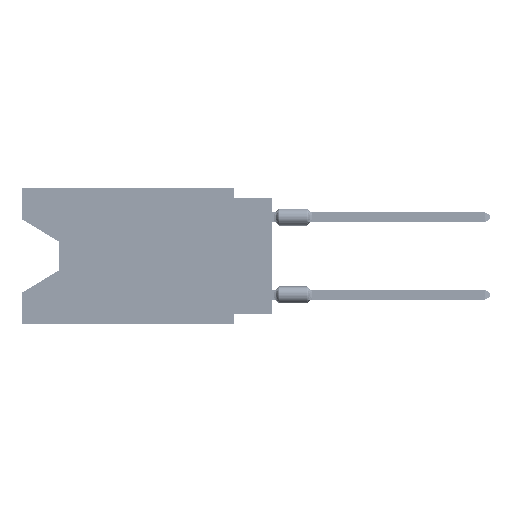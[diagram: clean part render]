
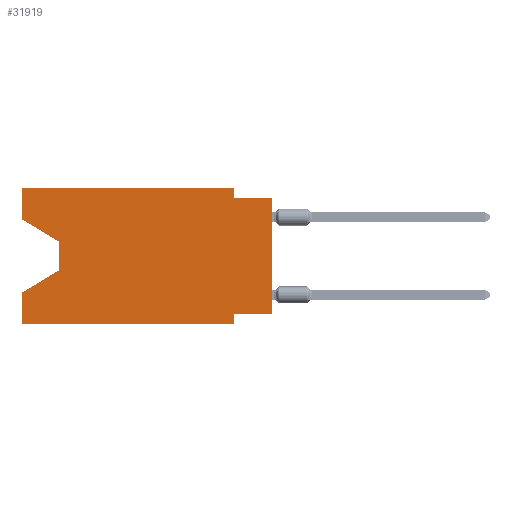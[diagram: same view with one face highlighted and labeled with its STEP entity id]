
A CAD part, left-side view. The second image highlights one B-rep face of the part: STEP entity #31919.
In plain terms, the highlighted planar face has unit normal (-1, 0, 0).
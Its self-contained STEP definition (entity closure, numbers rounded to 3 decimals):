
#1838 = AXIS2_PLACEMENT_3D ( 'NONE', #49395, #35175, #50359 ) ;
#1902 = EDGE_CURVE ( 'NONE', #17807, #44442, #88935, .T. ) ;
#2507 = VECTOR ( 'NONE', #56812, 1000. ) ;
#3308 = CARTESIAN_POINT ( 'NONE',  ( 0., 2.54, 0. ) ) ;
#3503 = VERTEX_POINT ( 'NONE', #51038 ) ;
#3532 = VECTOR ( 'NONE', #49575, 1000. ) ;
#3812 = CARTESIAN_POINT ( 'NONE',  ( 0., 16.383, -2.038 ) ) ;
#4411 = LINE ( 'NONE', #34366, #3532 ) ;
#4842 = VERTEX_POINT ( 'NONE', #69759 ) ;
#5623 = VECTOR ( 'NONE', #85334, 1000. ) ;
#6007 = LINE ( 'NONE', #35966, #92665 ) ;
#7443 = DIRECTION ( 'NONE',  ( 0., 0., -1. ) ) ;
#7530 = EDGE_CURVE ( 'NONE', #15331, #3503, #85624, .T. ) ;
#8111 = DIRECTION ( 'NONE',  ( 0., 0., -1. ) ) ;
#8975 = CARTESIAN_POINT ( 'NONE',  ( 0., 16.383, -6.852 ) ) ;
#10150 = CARTESIAN_POINT ( 'NONE',  ( 0., 0., -0.635 ) ) ;
#10381 = DIRECTION ( 'NONE',  ( 0., 1., 0. ) ) ;
#14312 = DIRECTION ( 'NONE',  ( 0., -1., 0. ) ) ;
#15331 = VERTEX_POINT ( 'NONE', #56127 ) ;
#16073 = VECTOR ( 'NONE', #48302, 1000. ) ;
#17807 = VERTEX_POINT ( 'NONE', #62234 ) ;
#19108 = EDGE_CURVE ( 'NONE', #44442, #82172, #93631, .T. ) ;
#19484 = PLANE ( 'NONE',  #1838 ) ;
#20814 = CARTESIAN_POINT ( 'NONE',  ( 0., 16.383, 0. ) ) ;
#20960 = CARTESIAN_POINT ( 'NONE',  ( 0., 16.383, -2.038 ) ) ;
#21267 = EDGE_LOOP ( 'NONE', ( #82074, #61064, #83660, #91899, #30325, #90696, #51275, #46634, #25352, #51942, #89945, #39362 ) ) ;
#23755 = EDGE_CURVE ( 'NONE', #66748, #15331, #47176, .T. ) ;
#24647 = CARTESIAN_POINT ( 'NONE',  ( 0., 13.97, -5.385 ) ) ;
#25352 = ORIENTED_EDGE ( 'NONE', *, *, #64418, .F. ) ;
#26879 = LINE ( 'NONE', #3812, #2507 ) ;
#28476 = EDGE_CURVE ( 'NONE', #66748, #57467, #29605, .T. ) ;
#28589 = DIRECTION ( 'NONE',  ( 0., 0., 1. ) ) ;
#28646 = VECTOR ( 'NONE', #14312, 1000. ) ;
#28647 = DIRECTION ( 'NONE',  ( 0., 0., 1. ) ) ;
#29263 = EDGE_CURVE ( 'NONE', #83175, #4842, #93589, .T. ) ;
#29605 = LINE ( 'NONE', #52175, #47051 ) ;
#30325 = ORIENTED_EDGE ( 'NONE', *, *, #90097, .T. ) ;
#30608 = CARTESIAN_POINT ( 'NONE',  ( 0., 16.383, 0. ) ) ;
#31919 = ADVANCED_FACE ( 'NONE', ( #48909 ), #19484, .F. ) ;
#34366 = CARTESIAN_POINT ( 'NONE',  ( 0., 16.383, -8.89 ) ) ;
#34486 = VECTOR ( 'NONE', #10381, 1000. ) ;
#35175 = DIRECTION ( 'NONE',  ( 1., 0., 0. ) ) ;
#35966 = CARTESIAN_POINT ( 'NONE',  ( 0., 16.383, 0. ) ) ;
#39065 = VECTOR ( 'NONE', #8111, 1000. ) ;
#39362 = ORIENTED_EDGE ( 'NONE', *, *, #63961, .F. ) ;
#41551 = EDGE_CURVE ( 'NONE', #74266, #17807, #26879, .T. ) ;
#44442 = VERTEX_POINT ( 'NONE', #24647 ) ;
#44731 = LINE ( 'NONE', #58010, #28646 ) ;
#45978 = DIRECTION ( 'NONE',  ( 0., -1., 0. ) ) ;
#46634 = ORIENTED_EDGE ( 'NONE', *, *, #28476, .T. ) ;
#47051 = VECTOR ( 'NONE', #67373, 1000. ) ;
#47176 = LINE ( 'NONE', #55051, #34486 ) ;
#47188 = VECTOR ( 'NONE', #45978, 1000. ) ;
#48302 = DIRECTION ( 'NONE',  ( 0., 0., -1. ) ) ;
#48909 = FACE_OUTER_BOUND ( 'NONE', #21267, .T. ) ;
#49395 = CARTESIAN_POINT ( 'NONE',  ( 0., 16.383, 0. ) ) ;
#49575 = DIRECTION ( 'NONE',  ( 0., -1., 0. ) ) ;
#50142 = VECTOR ( 'NONE', #28647, 1000. ) ;
#50249 = LINE ( 'NONE', #20814, #50142 ) ;
#50359 = DIRECTION ( 'NONE',  ( 0., 0., -1. ) ) ;
#51038 = CARTESIAN_POINT ( 'NONE',  ( 0., 2.54, -8.89 ) ) ;
#51128 = CARTESIAN_POINT ( 'NONE',  ( 0., 16.383, -8.89 ) ) ;
#51142 = VERTEX_POINT ( 'NONE', #30608 ) ;
#51275 = ORIENTED_EDGE ( 'NONE', *, *, #23755, .F. ) ;
#51942 = ORIENTED_EDGE ( 'NONE', *, *, #29263, .F. ) ;
#52175 = CARTESIAN_POINT ( 'NONE',  ( 0., 0., 0. ) ) ;
#55051 = CARTESIAN_POINT ( 'NONE',  ( 0., 0., -8.255 ) ) ;
#55748 = CARTESIAN_POINT ( 'NONE',  ( 0., 0., -0.635 ) ) ;
#56127 = CARTESIAN_POINT ( 'NONE',  ( 0., 2.54, -8.255 ) ) ;
#56812 = DIRECTION ( 'NONE',  ( 0., -0.855, -0.519 ) ) ;
#57467 = VERTEX_POINT ( 'NONE', #55748 ) ;
#58010 = CARTESIAN_POINT ( 'NONE',  ( 0., 16.383, 0. ) ) ;
#61064 = ORIENTED_EDGE ( 'NONE', *, *, #1902, .T. ) ;
#62234 = CARTESIAN_POINT ( 'NONE',  ( 0., 13.97, -3.505 ) ) ;
#62469 = EDGE_CURVE ( 'NONE', #69814, #82172, #50249, .T. ) ;
#63221 = CARTESIAN_POINT ( 'NONE',  ( 0., 13.97, -5.385 ) ) ;
#63961 = EDGE_CURVE ( 'NONE', #74266, #51142, #6007, .T. ) ;
#64418 = EDGE_CURVE ( 'NONE', #4842, #57467, #82809, .T. ) ;
#66548 = CARTESIAN_POINT ( 'NONE',  ( 0., 2.54, 0. ) ) ;
#66748 = VERTEX_POINT ( 'NONE', #73480 ) ;
#67373 = DIRECTION ( 'NONE',  ( 0., 0., 1. ) ) ;
#69759 = CARTESIAN_POINT ( 'NONE',  ( 0., 2.54, -0.635 ) ) ;
#69814 = VERTEX_POINT ( 'NONE', #51128 ) ;
#73480 = CARTESIAN_POINT ( 'NONE',  ( 0., 0., -8.255 ) ) ;
#74266 = VERTEX_POINT ( 'NONE', #20960 ) ;
#79214 = CARTESIAN_POINT ( 'NONE',  ( 0., 2.54, -8.89 ) ) ;
#80014 = EDGE_CURVE ( 'NONE', #51142, #83175, #44731, .T. ) ;
#82074 = ORIENTED_EDGE ( 'NONE', *, *, #41551, .T. ) ;
#82172 = VERTEX_POINT ( 'NONE', #8975 ) ;
#82809 = LINE ( 'NONE', #10150, #47188 ) ;
#83175 = VERTEX_POINT ( 'NONE', #3308 ) ;
#83660 = ORIENTED_EDGE ( 'NONE', *, *, #19108, .T. ) ;
#84462 = VECTOR ( 'NONE', #7443, 1000. ) ;
#85334 = DIRECTION ( 'NONE',  ( 0., 0.855, -0.519 ) ) ;
#85624 = LINE ( 'NONE', #79214, #16073 ) ;
#88935 = LINE ( 'NONE', #95805, #84462 ) ;
#89945 = ORIENTED_EDGE ( 'NONE', *, *, #80014, .F. ) ;
#90097 = EDGE_CURVE ( 'NONE', #69814, #3503, #4411, .T. ) ;
#90696 = ORIENTED_EDGE ( 'NONE', *, *, #7530, .F. ) ;
#91899 = ORIENTED_EDGE ( 'NONE', *, *, #62469, .F. ) ;
#92665 = VECTOR ( 'NONE', #28589, 1000. ) ;
#93589 = LINE ( 'NONE', #66548, #39065 ) ;
#93631 = LINE ( 'NONE', #63221, #5623 ) ;
#95805 = CARTESIAN_POINT ( 'NONE',  ( 0., 13.97, -3.505 ) ) ;
